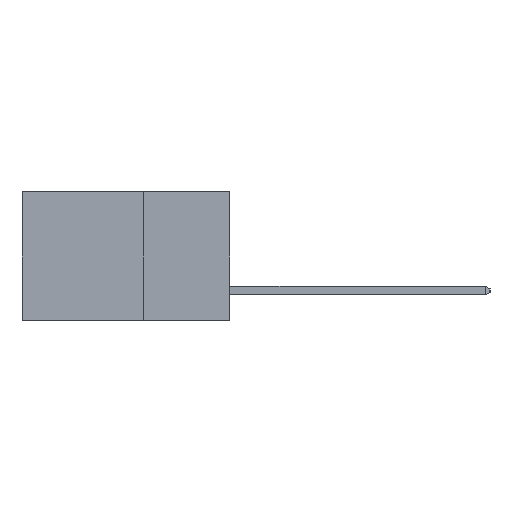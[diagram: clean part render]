
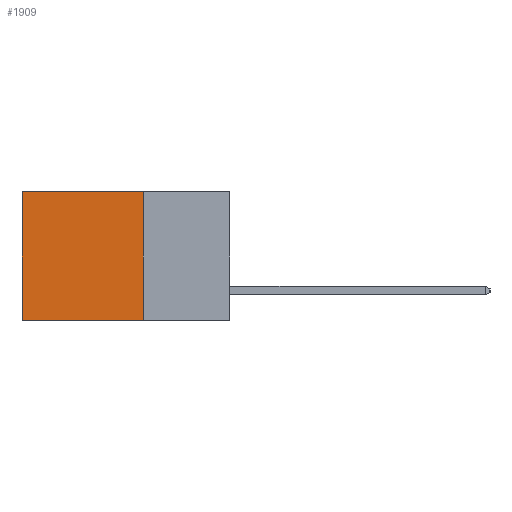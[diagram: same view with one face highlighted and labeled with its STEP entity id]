
A CAD part, left-side view. The second image highlights one B-rep face of the part: STEP entity #1909.
In plain terms, the highlighted planar face has unit normal (-1, 0, 0).
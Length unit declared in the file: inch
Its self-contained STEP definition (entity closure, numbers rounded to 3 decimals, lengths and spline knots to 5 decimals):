
#149 = VERTEX_POINT ( 'NONE', #12047 ) ;
#236 = VERTEX_POINT ( 'NONE', #10055 ) ;
#477 = VECTOR ( 'NONE', #5476, 39.37008 ) ;
#599 = VERTEX_POINT ( 'NONE', #2089 ) ;
#630 = CARTESIAN_POINT ( 'NONE',  ( 0.2615, 0.25, -0.37 ) ) ;
#640 = LINE ( 'NONE', #3983, #6148 ) ;
#1003 = EDGE_CURVE ( 'NONE', #236, #149, #3633, .T. ) ;
#1127 = EDGE_CURVE ( 'NONE', #12395, #236, #8462, .T. ) ;
#1909 = ADVANCED_FACE ( 'NONE', ( #6117 ), #12360, .F. ) ;
#2089 = CARTESIAN_POINT ( 'NONE',  ( 0.2615, 0.6, 0. ) ) ;
#3024 = ORIENTED_EDGE ( 'NONE', *, *, #1003, .F. ) ;
#3633 = LINE ( 'NONE', #630, #6164 ) ;
#3887 = DIRECTION ( 'NONE',  ( 0., 1., 0. ) ) ;
#3983 = CARTESIAN_POINT ( 'NONE',  ( 0.2615, 0.25, 0. ) ) ;
#4480 = AXIS2_PLACEMENT_3D ( 'NONE', #12314, #12301, #12298 ) ;
#4498 = DIRECTION ( 'NONE',  ( 0., 1., 0. ) ) ;
#4515 = ORIENTED_EDGE ( 'NONE', *, *, #11630, .T. ) ;
#4872 = LINE ( 'NONE', #6169, #7147 ) ;
#5476 = DIRECTION ( 'NONE',  ( 0., 0., -1. ) ) ;
#6117 = FACE_OUTER_BOUND ( 'NONE', #9375, .T. ) ;
#6148 = VECTOR ( 'NONE', #3887, 39.37008 ) ;
#6164 = VECTOR ( 'NONE', #4498, 39.37008 ) ;
#6169 = CARTESIAN_POINT ( 'NONE',  ( 0.2615, 0.6, -0.37 ) ) ;
#6206 = ORIENTED_EDGE ( 'NONE', *, *, #6765, .T. ) ;
#6765 = EDGE_CURVE ( 'NONE', #12395, #599, #640, .T. ) ;
#7147 = VECTOR ( 'NONE', #12416, 39.37008 ) ;
#7206 = ORIENTED_EDGE ( 'NONE', *, *, #1127, .F. ) ;
#8433 = CARTESIAN_POINT ( 'NONE',  ( 0.2615, 0.25, 0. ) ) ;
#8462 = LINE ( 'NONE', #9123, #477 ) ;
#9123 = CARTESIAN_POINT ( 'NONE',  ( 0.2615, 0.25, -0.37 ) ) ;
#9375 = EDGE_LOOP ( 'NONE', ( #4515, #3024, #7206, #6206 ) ) ;
#10055 = CARTESIAN_POINT ( 'NONE',  ( 0.2615, 0.25, -0.37 ) ) ;
#11630 = EDGE_CURVE ( 'NONE', #599, #149, #4872, .T. ) ;
#12047 = CARTESIAN_POINT ( 'NONE',  ( 0.2615, 0.6, -0.37 ) ) ;
#12298 = DIRECTION ( 'NONE',  ( 0., 0., -1. ) ) ;
#12301 = DIRECTION ( 'NONE',  ( 1., 0., 0. ) ) ;
#12314 = CARTESIAN_POINT ( 'NONE',  ( 0.2615, 0.25, -0.37 ) ) ;
#12360 = PLANE ( 'NONE',  #4480 ) ;
#12395 = VERTEX_POINT ( 'NONE', #8433 ) ;
#12416 = DIRECTION ( 'NONE',  ( 0., 0., -1. ) ) ;
